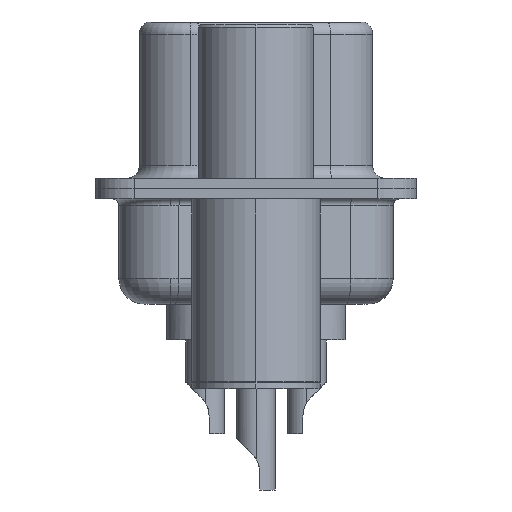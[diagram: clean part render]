
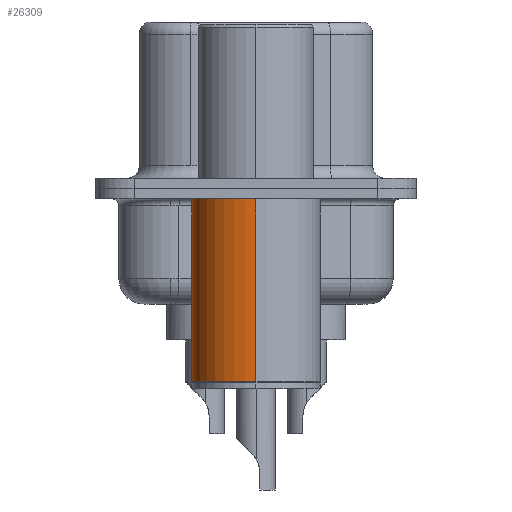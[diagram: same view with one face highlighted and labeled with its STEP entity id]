
A CAD part, left-side view. The second image highlights one B-rep face of the part: STEP entity #26309.
In plain terms, the highlighted cylindrical face has radius 2.5 mm (diameter 5 mm), a partial arc.
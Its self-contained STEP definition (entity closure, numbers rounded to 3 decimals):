
#727 = VERTEX_POINT ( 'NONE', #12620 ) ;
#1168 = CARTESIAN_POINT ( 'NONE',  ( 0., 0., -7.525 ) ) ;
#2317 = CARTESIAN_POINT ( 'NONE',  ( 0., 0., -0.4 ) ) ;
#3520 = DIRECTION ( 'NONE',  ( 1., 0., 0. ) ) ;
#3880 = EDGE_CURVE ( 'NONE', #6469, #727, #24417, .T. ) ;
#4286 = CIRCLE ( 'NONE', #27553, 2.5 ) ;
#4656 = DIRECTION ( 'NONE',  ( 1., 0., 0. ) ) ;
#5093 = CYLINDRICAL_SURFACE ( 'NONE', #11935, 2.5 ) ;
#5707 = ORIENTED_EDGE ( 'NONE', *, *, #28046, .T. ) ;
#5751 = CARTESIAN_POINT ( 'NONE',  ( 2.5, 0., -0.4 ) ) ;
#5783 = FACE_OUTER_BOUND ( 'NONE', #20033, .T. ) ;
#6289 = CARTESIAN_POINT ( 'NONE',  ( 2.5, 0., -7.525 ) ) ;
#6469 = VERTEX_POINT ( 'NONE', #9288 ) ;
#7506 = VECTOR ( 'NONE', #14975, 1000. ) ;
#8439 = EDGE_CURVE ( 'NONE', #26066, #727, #25391, .T. ) ;
#8802 = DIRECTION ( 'NONE',  ( 1., 0., 0. ) ) ;
#9288 = CARTESIAN_POINT ( 'NONE',  ( -2.5, 0., -7.525 ) ) ;
#9730 = VERTEX_POINT ( 'NONE', #6289 ) ;
#9866 = CARTESIAN_POINT ( 'NONE',  ( 2.5, 0., 0.581 ) ) ;
#11224 = LINE ( 'NONE', #9866, #11927 ) ;
#11927 = VECTOR ( 'NONE', #14327, 1000. ) ;
#11935 = AXIS2_PLACEMENT_3D ( 'NONE', #26354, #28461, #8802 ) ;
#12620 = CARTESIAN_POINT ( 'NONE',  ( -2.5, 0., -0.4 ) ) ;
#12935 = EDGE_CURVE ( 'NONE', #9730, #26066, #11224, .T. ) ;
#13165 = CARTESIAN_POINT ( 'NONE',  ( -2.5, 0., 0.581 ) ) ;
#13585 = AXIS2_PLACEMENT_3D ( 'NONE', #2317, #18027, #4656 ) ;
#14327 = DIRECTION ( 'NONE',  ( 0., 0., 1. ) ) ;
#14975 = DIRECTION ( 'NONE',  ( 0., 0., 1. ) ) ;
#16961 = DIRECTION ( 'NONE',  ( 0., 0., 1. ) ) ;
#18027 = DIRECTION ( 'NONE',  ( 0., 0., 1. ) ) ;
#18123 = ORIENTED_EDGE ( 'NONE', *, *, #12935, .F. ) ;
#18399 = ORIENTED_EDGE ( 'NONE', *, *, #3880, .T. ) ;
#20033 = EDGE_LOOP ( 'NONE', ( #5707, #18399, #23608, #18123 ) ) ;
#23608 = ORIENTED_EDGE ( 'NONE', *, *, #8439, .F. ) ;
#24417 = LINE ( 'NONE', #13165, #7506 ) ;
#25391 = CIRCLE ( 'NONE', #13585, 2.5 ) ;
#26066 = VERTEX_POINT ( 'NONE', #5751 ) ;
#26309 = ADVANCED_FACE ( 'NONE', ( #5783 ), #5093, .T. ) ;
#26354 = CARTESIAN_POINT ( 'NONE',  ( 0., 0., 0.581 ) ) ;
#27553 = AXIS2_PLACEMENT_3D ( 'NONE', #1168, #16961, #3520 ) ;
#28046 = EDGE_CURVE ( 'NONE', #9730, #6469, #4286, .T. ) ;
#28461 = DIRECTION ( 'NONE',  ( 0., 0., 1. ) ) ;
